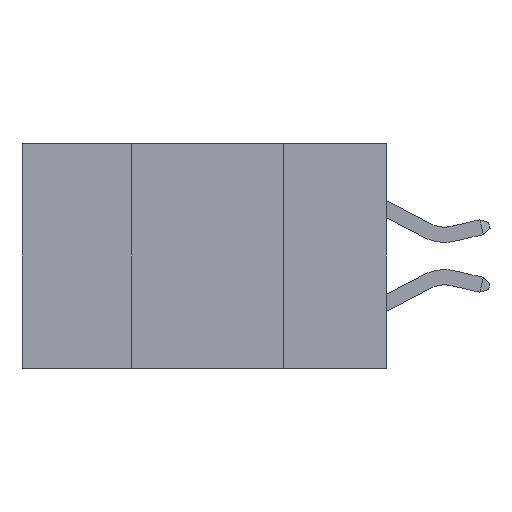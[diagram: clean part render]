
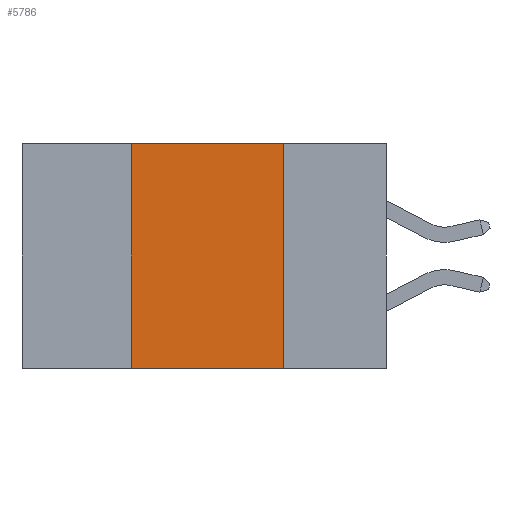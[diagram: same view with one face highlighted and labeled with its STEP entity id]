
A CAD part, left-side view. The second image highlights one B-rep face of the part: STEP entity #5786.
In plain terms, the highlighted planar face has unit normal (-1, 0, 0).
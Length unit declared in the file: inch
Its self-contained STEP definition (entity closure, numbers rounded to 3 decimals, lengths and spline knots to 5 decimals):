
#709 = DIRECTION ( 'NONE',  ( 1., 0., 0. ) ) ;
#921 = LINE ( 'NONE', #13945, #11560 ) ;
#1153 = CARTESIAN_POINT ( 'NONE',  ( 0., 0.17, -0.37 ) ) ;
#1193 = DIRECTION ( 'NONE',  ( 0., 0., 1. ) ) ;
#1281 = EDGE_CURVE ( 'NONE', #8936, #10585, #14868, .T. ) ;
#1981 = VECTOR ( 'NONE', #1193, 39.37008 ) ;
#2930 = AXIS2_PLACEMENT_3D ( 'NONE', #12207, #709, #10919 ) ;
#2935 = FACE_OUTER_BOUND ( 'NONE', #13632, .T. ) ;
#3311 = EDGE_CURVE ( 'NONE', #3534, #10585, #921, .T. ) ;
#3534 = VERTEX_POINT ( 'NONE', #7442 ) ;
#3617 = LINE ( 'NONE', #12840, #1981 ) ;
#3644 = DIRECTION ( 'NONE',  ( 0., -1., 0. ) ) ;
#3900 = VERTEX_POINT ( 'NONE', #11085 ) ;
#4415 = ORIENTED_EDGE ( 'NONE', *, *, #13057, .F. ) ;
#4469 = DIRECTION ( 'NONE',  ( 0., -1., 0. ) ) ;
#5786 = ADVANCED_FACE ( 'NONE', ( #2935 ), #14586, .F. ) ;
#5818 = VECTOR ( 'NONE', #3644, 39.37008 ) ;
#6153 = VECTOR ( 'NONE', #8374, 39.37008 ) ;
#6222 = CARTESIAN_POINT ( 'NONE',  ( 0., 0.17, 0. ) ) ;
#6931 = ORIENTED_EDGE ( 'NONE', *, *, #3311, .T. ) ;
#7442 = CARTESIAN_POINT ( 'NONE',  ( 0., 0.42, -0.37 ) ) ;
#8374 = DIRECTION ( 'NONE',  ( 0., 0., -1. ) ) ;
#8936 = VERTEX_POINT ( 'NONE', #6222 ) ;
#8941 = ORIENTED_EDGE ( 'NONE', *, *, #1281, .F. ) ;
#9631 = EDGE_CURVE ( 'NONE', #3900, #8936, #13022, .T. ) ;
#10585 = VERTEX_POINT ( 'NONE', #14731 ) ;
#10919 = DIRECTION ( 'NONE',  ( 0., 0., -1. ) ) ;
#11085 = CARTESIAN_POINT ( 'NONE',  ( 0., 0.42, 0. ) ) ;
#11560 = VECTOR ( 'NONE', #4469, 39.37008 ) ;
#11864 = CARTESIAN_POINT ( 'NONE',  ( 0., 0.6, 0. ) ) ;
#12207 = CARTESIAN_POINT ( 'NONE',  ( 0., 0.6, 0. ) ) ;
#12840 = CARTESIAN_POINT ( 'NONE',  ( 0., 0.42, -0.37 ) ) ;
#13022 = LINE ( 'NONE', #11864, #5818 ) ;
#13057 = EDGE_CURVE ( 'NONE', #3534, #3900, #3617, .T. ) ;
#13632 = EDGE_LOOP ( 'NONE', ( #8941, #14452, #4415, #6931 ) ) ;
#13945 = CARTESIAN_POINT ( 'NONE',  ( 0., 0.6, -0.37 ) ) ;
#14452 = ORIENTED_EDGE ( 'NONE', *, *, #9631, .F. ) ;
#14586 = PLANE ( 'NONE',  #2930 ) ;
#14731 = CARTESIAN_POINT ( 'NONE',  ( 0., 0.17, -0.37 ) ) ;
#14868 = LINE ( 'NONE', #1153, #6153 ) ;
